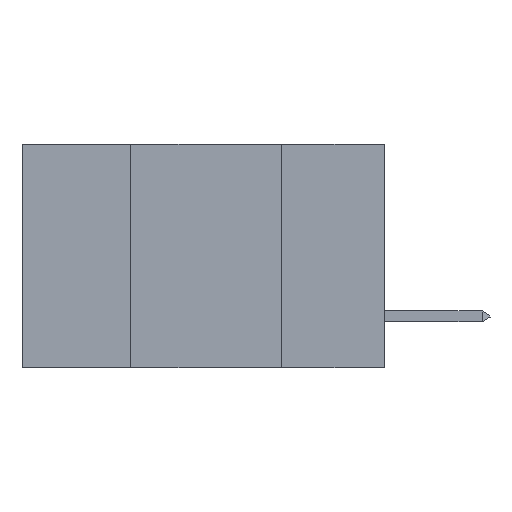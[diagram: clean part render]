
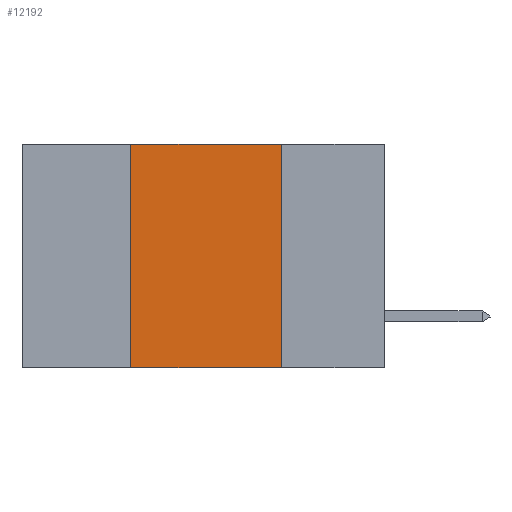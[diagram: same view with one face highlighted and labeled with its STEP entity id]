
A CAD part, left-side view. The second image highlights one B-rep face of the part: STEP entity #12192.
In plain terms, the highlighted planar face has unit normal (-1, 0, 0).
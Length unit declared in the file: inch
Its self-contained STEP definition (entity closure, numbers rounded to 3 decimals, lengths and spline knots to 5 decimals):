
#125 = VECTOR ( 'NONE', #13389, 39.37008 ) ;
#618 = CARTESIAN_POINT ( 'NONE',  ( 0., 0.17, 0. ) ) ;
#1129 = VERTEX_POINT ( 'NONE', #1885 ) ;
#1403 = EDGE_CURVE ( 'NONE', #1698, #1129, #5422, .T. ) ;
#1602 = EDGE_CURVE ( 'NONE', #1698, #9841, #4759, .T. ) ;
#1698 = VERTEX_POINT ( 'NONE', #14426 ) ;
#1825 = ORIENTED_EDGE ( 'NONE', *, *, #1403, .T. ) ;
#1855 = EDGE_CURVE ( 'NONE', #5288, #1129, #11520, .T. ) ;
#1885 = CARTESIAN_POINT ( 'NONE',  ( 0., 0.17, -0.37 ) ) ;
#2421 = PLANE ( 'NONE',  #12726 ) ;
#3059 = EDGE_CURVE ( 'NONE', #9841, #5288, #17272, .T. ) ;
#3863 = DIRECTION ( 'NONE',  ( 0., -1., 0. ) ) ;
#4759 = LINE ( 'NONE', #9995, #15837 ) ;
#4873 = CARTESIAN_POINT ( 'NONE',  ( 0., 0.17, 0. ) ) ;
#5288 = VERTEX_POINT ( 'NONE', #4873 ) ;
#5324 = DIRECTION ( 'NONE',  ( 1., 0., 0. ) ) ;
#5422 = LINE ( 'NONE', #13649, #9130 ) ;
#5762 = CARTESIAN_POINT ( 'NONE',  ( 0., 0.42, 0. ) ) ;
#6452 = CARTESIAN_POINT ( 'NONE',  ( 0., 0.6, 0. ) ) ;
#7609 = ORIENTED_EDGE ( 'NONE', *, *, #1602, .F. ) ;
#9130 = VECTOR ( 'NONE', #3863, 39.37008 ) ;
#9841 = VERTEX_POINT ( 'NONE', #5762 ) ;
#9948 = FACE_OUTER_BOUND ( 'NONE', #15693, .T. ) ;
#9995 = CARTESIAN_POINT ( 'NONE',  ( 0., 0.42, 0. ) ) ;
#10467 = ORIENTED_EDGE ( 'NONE', *, *, #3059, .F. ) ;
#11520 = LINE ( 'NONE', #618, #125 ) ;
#12192 = ADVANCED_FACE ( 'NONE', ( #9948 ), #2421, .F. ) ;
#12726 = AXIS2_PLACEMENT_3D ( 'NONE', #13669, #5324, #15064 ) ;
#13282 = ORIENTED_EDGE ( 'NONE', *, *, #1855, .F. ) ;
#13389 = DIRECTION ( 'NONE',  ( 0., 0., -1. ) ) ;
#13641 = VECTOR ( 'NONE', #17486, 39.37008 ) ;
#13649 = CARTESIAN_POINT ( 'NONE',  ( 0., 0.6, -0.37 ) ) ;
#13669 = CARTESIAN_POINT ( 'NONE',  ( 0., 0.6, 0. ) ) ;
#14194 = DIRECTION ( 'NONE',  ( 0., 0., 1. ) ) ;
#14426 = CARTESIAN_POINT ( 'NONE',  ( 0., 0.42, -0.37 ) ) ;
#15064 = DIRECTION ( 'NONE',  ( 0., 0., -1. ) ) ;
#15693 = EDGE_LOOP ( 'NONE', ( #13282, #10467, #7609, #1825 ) ) ;
#15837 = VECTOR ( 'NONE', #14194, 39.37008 ) ;
#17272 = LINE ( 'NONE', #6452, #13641 ) ;
#17486 = DIRECTION ( 'NONE',  ( 0., -1., 0. ) ) ;
